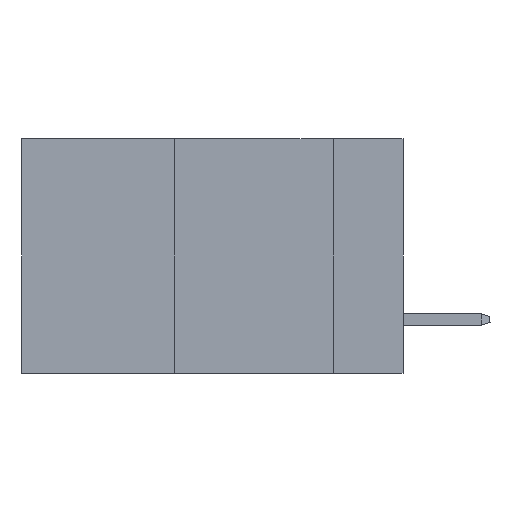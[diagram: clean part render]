
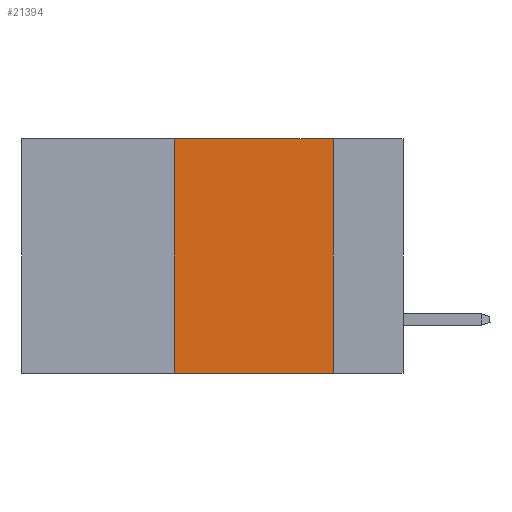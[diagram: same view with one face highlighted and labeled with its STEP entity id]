
A CAD part, left-side view. The second image highlights one B-rep face of the part: STEP entity #21394.
In plain terms, the highlighted planar face has unit normal (-1, 0, 0).
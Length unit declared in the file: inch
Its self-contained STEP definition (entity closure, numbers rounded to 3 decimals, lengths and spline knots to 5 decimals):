
#147 = EDGE_CURVE ( 'NONE', #700, #21826, #11037, .T. ) ;
#700 = VERTEX_POINT ( 'NONE', #15303 ) ;
#852 = EDGE_CURVE ( 'NONE', #700, #8748, #14185, .T. ) ;
#1765 = VECTOR ( 'NONE', #5557, 39.37008 ) ;
#2233 = DIRECTION ( 'NONE',  ( 0., 0., -1. ) ) ;
#2827 = CARTESIAN_POINT ( 'NONE',  ( 0., 0.11, -0.37 ) ) ;
#3736 = ORIENTED_EDGE ( 'NONE', *, *, #21395, .F. ) ;
#4441 = CARTESIAN_POINT ( 'NONE',  ( 0., 0.11, 0. ) ) ;
#4812 = DIRECTION ( 'NONE',  ( 0., -1., 0. ) ) ;
#4869 = VECTOR ( 'NONE', #4812, 39.37008 ) ;
#4971 = EDGE_LOOP ( 'NONE', ( #3736, #23436, #16425, #22001 ) ) ;
#5557 = DIRECTION ( 'NONE',  ( 0., -1., 0. ) ) ;
#6538 = VECTOR ( 'NONE', #24356, 39.37008 ) ;
#6800 = CARTESIAN_POINT ( 'NONE',  ( 0., 0.6, -0.37 ) ) ;
#8163 = DIRECTION ( 'NONE',  ( 0., 0., -1. ) ) ;
#8422 = VECTOR ( 'NONE', #8163, 39.37008 ) ;
#8748 = VERTEX_POINT ( 'NONE', #2827 ) ;
#9277 = CARTESIAN_POINT ( 'NONE',  ( 0., 0.11, 0. ) ) ;
#10079 = CARTESIAN_POINT ( 'NONE',  ( 0., 0.36, 0. ) ) ;
#11037 = LINE ( 'NONE', #24109, #6538 ) ;
#11716 = DIRECTION ( 'NONE',  ( 1., 0., 0. ) ) ;
#12324 = VERTEX_POINT ( 'NONE', #9277 ) ;
#12950 = LINE ( 'NONE', #16995, #1765 ) ;
#13077 = FACE_OUTER_BOUND ( 'NONE', #4971, .T. ) ;
#14185 = LINE ( 'NONE', #6800, #4869 ) ;
#14607 = EDGE_CURVE ( 'NONE', #21826, #12324, #12950, .T. ) ;
#15303 = CARTESIAN_POINT ( 'NONE',  ( 0., 0.36, -0.37 ) ) ;
#15408 = LINE ( 'NONE', #4441, #8422 ) ;
#15772 = CARTESIAN_POINT ( 'NONE',  ( 0., 0.6, 0. ) ) ;
#16425 = ORIENTED_EDGE ( 'NONE', *, *, #147, .F. ) ;
#16995 = CARTESIAN_POINT ( 'NONE',  ( 0., 0.6, 0. ) ) ;
#17054 = AXIS2_PLACEMENT_3D ( 'NONE', #15772, #11716, #2233 ) ;
#20607 = PLANE ( 'NONE',  #17054 ) ;
#21394 = ADVANCED_FACE ( 'NONE', ( #13077 ), #20607, .F. ) ;
#21395 = EDGE_CURVE ( 'NONE', #12324, #8748, #15408, .T. ) ;
#21826 = VERTEX_POINT ( 'NONE', #10079 ) ;
#22001 = ORIENTED_EDGE ( 'NONE', *, *, #852, .T. ) ;
#23436 = ORIENTED_EDGE ( 'NONE', *, *, #14607, .F. ) ;
#24109 = CARTESIAN_POINT ( 'NONE',  ( 0., 0.36, 0. ) ) ;
#24356 = DIRECTION ( 'NONE',  ( 0., 0., 1. ) ) ;
